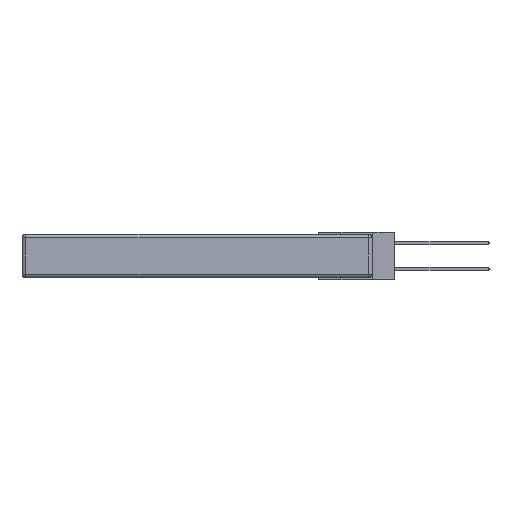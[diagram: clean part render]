
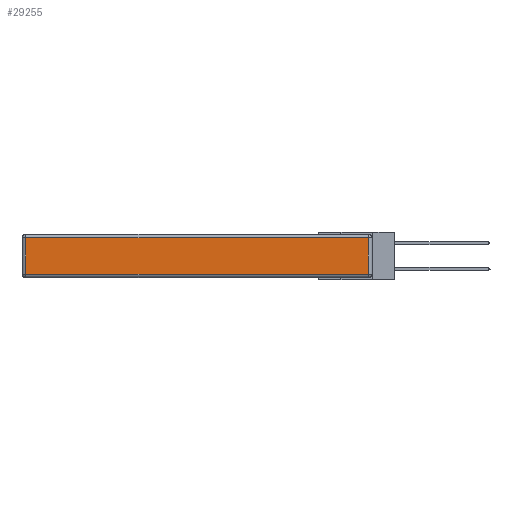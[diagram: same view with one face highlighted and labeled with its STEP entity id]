
A CAD part, left-side view. The second image highlights one B-rep face of the part: STEP entity #29255.
In plain terms, the highlighted planar face has unit normal (-1, 0, 0).
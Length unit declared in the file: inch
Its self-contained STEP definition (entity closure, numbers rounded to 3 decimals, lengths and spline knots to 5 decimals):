
#233 = VECTOR ( 'NONE', #16583, 39.37008 ) ;
#552 = CARTESIAN_POINT ( 'NONE',  ( 0., 2.72, -0.343 ) ) ;
#733 = AXIS2_PLACEMENT_3D ( 'NONE', #5738, #24204, #8339 ) ;
#1767 = VERTEX_POINT ( 'NONE', #19953 ) ;
#2566 = EDGE_CURVE ( 'NONE', #1767, #12538, #25637, .T. ) ;
#5288 = PLANE ( 'NONE',  #733 ) ;
#5738 = CARTESIAN_POINT ( 'NONE',  ( 0., 0., -0.343 ) ) ;
#5948 = EDGE_CURVE ( 'NONE', #18936, #7577, #6351, .T. ) ;
#6066 = CARTESIAN_POINT ( 'NONE',  ( 0., 0., -0.313 ) ) ;
#6351 = LINE ( 'NONE', #6066, #33636 ) ;
#6828 = DIRECTION ( 'NONE',  ( 0., 0., 1. ) ) ;
#7005 = VECTOR ( 'NONE', #12613, 39.37008 ) ;
#7577 = VERTEX_POINT ( 'NONE', #20496 ) ;
#8339 = DIRECTION ( 'NONE',  ( 0., 0., 1. ) ) ;
#11176 = FACE_OUTER_BOUND ( 'NONE', #19721, .T. ) ;
#11281 = EDGE_CURVE ( 'NONE', #7577, #1767, #16955, .T. ) ;
#12538 = VERTEX_POINT ( 'NONE', #33224 ) ;
#12613 = DIRECTION ( 'NONE',  ( 0., 1., 0. ) ) ;
#14906 = VECTOR ( 'NONE', #6828, 39.37008 ) ;
#16583 = DIRECTION ( 'NONE',  ( 0., 0., -1. ) ) ;
#16955 = LINE ( 'NONE', #17101, #14906 ) ;
#17101 = CARTESIAN_POINT ( 'NONE',  ( 0., 0.03, -0.343 ) ) ;
#17705 = CARTESIAN_POINT ( 'NONE',  ( 0., 2.75, -0.03 ) ) ;
#18936 = VERTEX_POINT ( 'NONE', #24402 ) ;
#19313 = ORIENTED_EDGE ( 'NONE', *, *, #20723, .T. ) ;
#19334 = ORIENTED_EDGE ( 'NONE', *, *, #2566, .T. ) ;
#19721 = EDGE_LOOP ( 'NONE', ( #32465, #19743, #19334, #19313 ) ) ;
#19743 = ORIENTED_EDGE ( 'NONE', *, *, #11281, .T. ) ;
#19953 = CARTESIAN_POINT ( 'NONE',  ( 0., 0.03, -0.03 ) ) ;
#20496 = CARTESIAN_POINT ( 'NONE',  ( 0., 0.03, -0.313 ) ) ;
#20723 = EDGE_CURVE ( 'NONE', #12538, #18936, #34143, .T. ) ;
#20758 = DIRECTION ( 'NONE',  ( 0., -1., 0. ) ) ;
#24204 = DIRECTION ( 'NONE',  ( -1., 0., 0. ) ) ;
#24402 = CARTESIAN_POINT ( 'NONE',  ( 0., 2.72, -0.313 ) ) ;
#25637 = LINE ( 'NONE', #17705, #7005 ) ;
#29255 = ADVANCED_FACE ( 'NONE', ( #11176 ), #5288, .T. ) ;
#32465 = ORIENTED_EDGE ( 'NONE', *, *, #5948, .T. ) ;
#33224 = CARTESIAN_POINT ( 'NONE',  ( 0., 2.72, -0.03 ) ) ;
#33636 = VECTOR ( 'NONE', #20758, 39.37008 ) ;
#34143 = LINE ( 'NONE', #552, #233 ) ;
